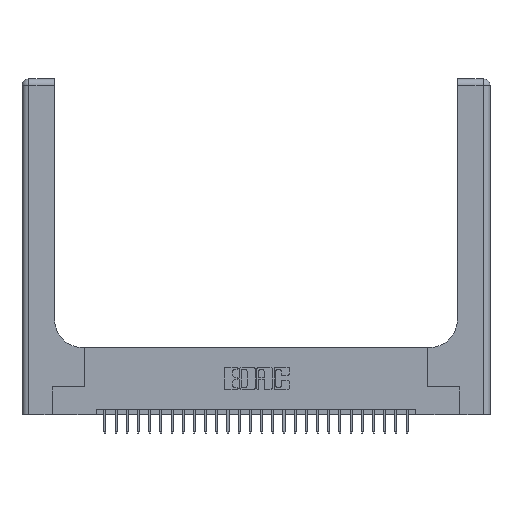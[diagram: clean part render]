
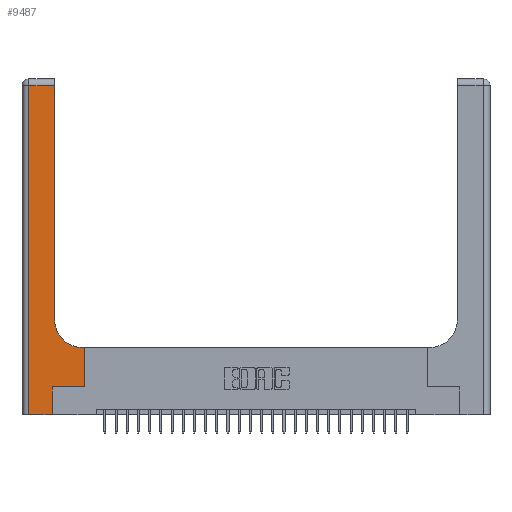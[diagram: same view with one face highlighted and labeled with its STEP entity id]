
A CAD part, top view. The second image highlights one B-rep face of the part: STEP entity #9487.
In plain terms, the highlighted planar face has unit normal (0, 0, 1).
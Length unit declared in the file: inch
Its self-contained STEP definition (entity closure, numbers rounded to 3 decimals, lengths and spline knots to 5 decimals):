
#62 = LINE ( 'NONE', #27041, #764 ) ;
#386 = CARTESIAN_POINT ( 'NONE',  ( 0.5585, 0.6, 0.37 ) ) ;
#398 = DIRECTION ( 'NONE',  ( 0., 0., -1. ) ) ;
#724 = LINE ( 'NONE', #3151, #23965 ) ;
#764 = VECTOR ( 'NONE', #13569, 39.37008 ) ;
#1186 = VECTOR ( 'NONE', #24273, 39.37008 ) ;
#1199 = VERTEX_POINT ( 'NONE', #22892 ) ;
#1430 = DIRECTION ( 'NONE',  ( 0., 1., 0. ) ) ;
#1547 = VERTEX_POINT ( 'NONE', #28550 ) ;
#1660 = DIRECTION ( 'NONE',  ( 1., 0., 0. ) ) ;
#3146 = EDGE_CURVE ( 'NONE', #1199, #28556, #62, .T. ) ;
#3151 = CARTESIAN_POINT ( 'NONE',  ( 0.06, 3., 0.37 ) ) ;
#3209 = VECTOR ( 'NONE', #1660, 39.37008 ) ;
#4119 = CARTESIAN_POINT ( 'NONE',  ( 0.2915, 0.6, 0.37 ) ) ;
#4184 = ORIENTED_EDGE ( 'NONE', *, *, #13028, .T. ) ;
#5284 = VERTEX_POINT ( 'NONE', #12296 ) ;
#6843 = VECTOR ( 'NONE', #25287, 39.37008 ) ;
#7708 = VECTOR ( 'NONE', #11583, 39.37008 ) ;
#8207 = CARTESIAN_POINT ( 'NONE',  ( 0.269, 0., 0.37 ) ) ;
#8336 = CARTESIAN_POINT ( 'NONE',  ( 0., 0., 0.37 ) ) ;
#9487 = ADVANCED_FACE ( 'NONE', ( #9782 ), #13859, .F. ) ;
#9782 = FACE_OUTER_BOUND ( 'NONE', #11106, .T. ) ;
#10808 = VERTEX_POINT ( 'NONE', #23156 ) ;
#11106 = EDGE_LOOP ( 'NONE', ( #14033, #22929, #28587, #12420, #4184, #20719, #23144, #16394, #12377 ) ) ;
#11271 = VERTEX_POINT ( 'NONE', #26836 ) ;
#11389 = DIRECTION ( 'NONE',  ( 0., 0., -1. ) ) ;
#11583 = DIRECTION ( 'NONE',  ( -1., 0., 0. ) ) ;
#12296 = CARTESIAN_POINT ( 'NONE',  ( 0.269, 0., 0.37 ) ) ;
#12377 = ORIENTED_EDGE ( 'NONE', *, *, #13821, .T. ) ;
#12420 = ORIENTED_EDGE ( 'NONE', *, *, #14154, .T. ) ;
#13028 = EDGE_CURVE ( 'NONE', #5284, #1199, #14870, .T. ) ;
#13149 = LINE ( 'NONE', #4119, #1186 ) ;
#13569 = DIRECTION ( 'NONE',  ( 1., 0., 0. ) ) ;
#13654 = LINE ( 'NONE', #27278, #7708 ) ;
#13757 = CARTESIAN_POINT ( 'NONE',  ( 0., 3., 0.37 ) ) ;
#13787 = AXIS2_PLACEMENT_3D ( 'NONE', #24847, #11389, #27090 ) ;
#13821 = EDGE_CURVE ( 'NONE', #10808, #11271, #28906, .T. ) ;
#13859 = PLANE ( 'NONE',  #19601 ) ;
#14033 = ORIENTED_EDGE ( 'NONE', *, *, #27381, .T. ) ;
#14154 = EDGE_CURVE ( 'NONE', #27297, #5284, #15152, .T. ) ;
#14870 = LINE ( 'NONE', #8207, #19474 ) ;
#15152 = LINE ( 'NONE', #8336, #3209 ) ;
#16109 = DIRECTION ( 'NONE',  ( -1., 0., 0. ) ) ;
#16394 = ORIENTED_EDGE ( 'NONE', *, *, #18412, .T. ) ;
#16580 = DIRECTION ( 'NONE',  ( 0., -1., 0. ) ) ;
#16837 = CARTESIAN_POINT ( 'NONE',  ( 0.06, 0., 0.37 ) ) ;
#17016 = LINE ( 'NONE', #19227, #27551 ) ;
#17480 = EDGE_CURVE ( 'NONE', #28556, #19918, #24060, .T. ) ;
#18412 = EDGE_CURVE ( 'NONE', #19918, #10808, #13149, .T. ) ;
#18568 = VERTEX_POINT ( 'NONE', #27087 ) ;
#19227 = CARTESIAN_POINT ( 'NONE',  ( 0.2915, 3., 0.37 ) ) ;
#19333 = DIRECTION ( 'NONE',  ( 0., 1., 0. ) ) ;
#19474 = VECTOR ( 'NONE', #1430, 39.37008 ) ;
#19601 = AXIS2_PLACEMENT_3D ( 'NONE', #13757, #398, #16109 ) ;
#19918 = VERTEX_POINT ( 'NONE', #386 ) ;
#20055 = EDGE_CURVE ( 'NONE', #18568, #27297, #724, .T. ) ;
#20719 = ORIENTED_EDGE ( 'NONE', *, *, #3146, .T. ) ;
#21144 = CARTESIAN_POINT ( 'NONE',  ( 0.5585, 0.25, 0.37 ) ) ;
#22892 = CARTESIAN_POINT ( 'NONE',  ( 0.269, 0.25, 0.37 ) ) ;
#22929 = ORIENTED_EDGE ( 'NONE', *, *, #24741, .T. ) ;
#23048 = CARTESIAN_POINT ( 'NONE',  ( 0.5585, 0.25, 0.37 ) ) ;
#23144 = ORIENTED_EDGE ( 'NONE', *, *, #17480, .T. ) ;
#23156 = CARTESIAN_POINT ( 'NONE',  ( 0.5415, 0.6, 0.37 ) ) ;
#23965 = VECTOR ( 'NONE', #16580, 39.37008 ) ;
#24060 = LINE ( 'NONE', #23048, #6843 ) ;
#24273 = DIRECTION ( 'NONE',  ( -1., 0., 0. ) ) ;
#24741 = EDGE_CURVE ( 'NONE', #1547, #18568, #13654, .T. ) ;
#24847 = CARTESIAN_POINT ( 'NONE',  ( 0.5415, 0.85, 0.37 ) ) ;
#25287 = DIRECTION ( 'NONE',  ( 0., 1., 0. ) ) ;
#26836 = CARTESIAN_POINT ( 'NONE',  ( 0.2915, 0.85, 0.37 ) ) ;
#27041 = CARTESIAN_POINT ( 'NONE',  ( 0.269, 0.25, 0.37 ) ) ;
#27087 = CARTESIAN_POINT ( 'NONE',  ( 0.06, 2.94, 0.37 ) ) ;
#27090 = DIRECTION ( 'NONE',  ( 1., 0., 0. ) ) ;
#27278 = CARTESIAN_POINT ( 'NONE',  ( 0., 2.94, 0.37 ) ) ;
#27297 = VERTEX_POINT ( 'NONE', #16837 ) ;
#27381 = EDGE_CURVE ( 'NONE', #11271, #1547, #17016, .T. ) ;
#27551 = VECTOR ( 'NONE', #19333, 39.37008 ) ;
#28550 = CARTESIAN_POINT ( 'NONE',  ( 0.2915, 2.94, 0.37 ) ) ;
#28556 = VERTEX_POINT ( 'NONE', #21144 ) ;
#28587 = ORIENTED_EDGE ( 'NONE', *, *, #20055, .T. ) ;
#28906 = CIRCLE ( 'NONE', #13787, 0.25 ) ;
